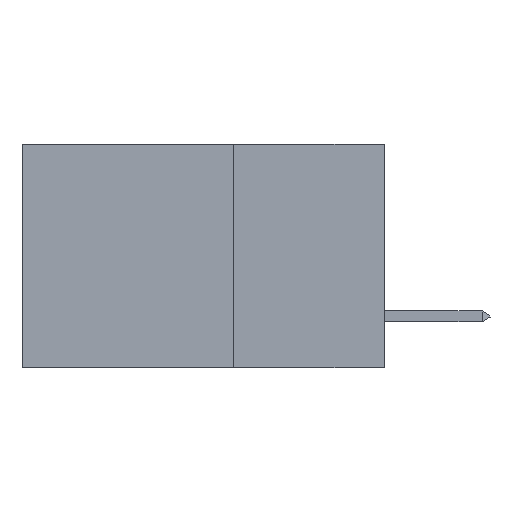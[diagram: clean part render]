
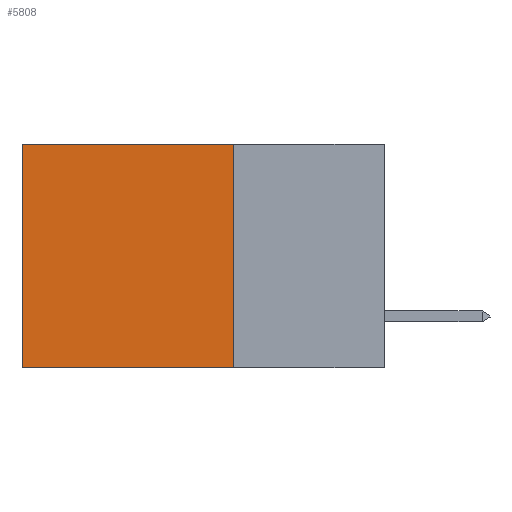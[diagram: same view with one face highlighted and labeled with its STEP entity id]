
A CAD part, left-side view. The second image highlights one B-rep face of the part: STEP entity #5808.
In plain terms, the highlighted planar face has unit normal (-1, 0, 0).
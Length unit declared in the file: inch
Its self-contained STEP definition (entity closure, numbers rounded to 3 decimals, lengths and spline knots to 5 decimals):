
#381 = LINE ( 'NONE', #2334, #2680 ) ;
#2334 = CARTESIAN_POINT ( 'NONE',  ( 0.2875, 0.25, 0. ) ) ;
#2680 = VECTOR ( 'NONE', #3380, 39.37008 ) ;
#3380 = DIRECTION ( 'NONE',  ( 0., 1., 0. ) ) ;
#3557 = EDGE_CURVE ( 'NONE', #10794, #9074, #14118, .T. ) ;
#3626 = CARTESIAN_POINT ( 'NONE',  ( 0.2875, 0.25, -0.37 ) ) ;
#3853 = VECTOR ( 'NONE', #5760, 39.37008 ) ;
#4007 = LINE ( 'NONE', #13145, #9367 ) ;
#4405 = CARTESIAN_POINT ( 'NONE',  ( 0.2875, 0.25, -0.37 ) ) ;
#4545 = LINE ( 'NONE', #9383, #3853 ) ;
#4831 = ORIENTED_EDGE ( 'NONE', *, *, #13542, .F. ) ;
#5714 = EDGE_CURVE ( 'NONE', #8551, #14128, #381, .T. ) ;
#5760 = DIRECTION ( 'NONE',  ( 0., 0., -1. ) ) ;
#5808 = ADVANCED_FACE ( 'NONE', ( #6712 ), #7365, .F. ) ;
#5814 = DIRECTION ( 'NONE',  ( 0., 1., 0. ) ) ;
#5963 = ORIENTED_EDGE ( 'NONE', *, *, #5714, .T. ) ;
#6712 = FACE_OUTER_BOUND ( 'NONE', #7795, .T. ) ;
#6905 = VECTOR ( 'NONE', #5814, 39.37008 ) ;
#7346 = CARTESIAN_POINT ( 'NONE',  ( 0.2875, 0.6, 0. ) ) ;
#7365 = PLANE ( 'NONE',  #7660 ) ;
#7518 = DIRECTION ( 'NONE',  ( 1., 0., 0. ) ) ;
#7660 = AXIS2_PLACEMENT_3D ( 'NONE', #11913, #7518, #9600 ) ;
#7795 = EDGE_LOOP ( 'NONE', ( #13125, #13620, #4831, #5963 ) ) ;
#8551 = VERTEX_POINT ( 'NONE', #13695 ) ;
#8714 = EDGE_CURVE ( 'NONE', #14128, #9074, #4007, .T. ) ;
#9074 = VERTEX_POINT ( 'NONE', #9871 ) ;
#9367 = VECTOR ( 'NONE', #10887, 39.37008 ) ;
#9383 = CARTESIAN_POINT ( 'NONE',  ( 0.2875, 0.25, 0. ) ) ;
#9600 = DIRECTION ( 'NONE',  ( 0., 0., -1. ) ) ;
#9871 = CARTESIAN_POINT ( 'NONE',  ( 0.2875, 0.6, -0.37 ) ) ;
#10794 = VERTEX_POINT ( 'NONE', #4405 ) ;
#10887 = DIRECTION ( 'NONE',  ( 0., 0., -1. ) ) ;
#11913 = CARTESIAN_POINT ( 'NONE',  ( 0.2875, 0.25, 0. ) ) ;
#13125 = ORIENTED_EDGE ( 'NONE', *, *, #8714, .T. ) ;
#13145 = CARTESIAN_POINT ( 'NONE',  ( 0.2875, 0.6, 0. ) ) ;
#13542 = EDGE_CURVE ( 'NONE', #8551, #10794, #4545, .T. ) ;
#13620 = ORIENTED_EDGE ( 'NONE', *, *, #3557, .F. ) ;
#13695 = CARTESIAN_POINT ( 'NONE',  ( 0.2875, 0.25, 0. ) ) ;
#14118 = LINE ( 'NONE', #3626, #6905 ) ;
#14128 = VERTEX_POINT ( 'NONE', #7346 ) ;
